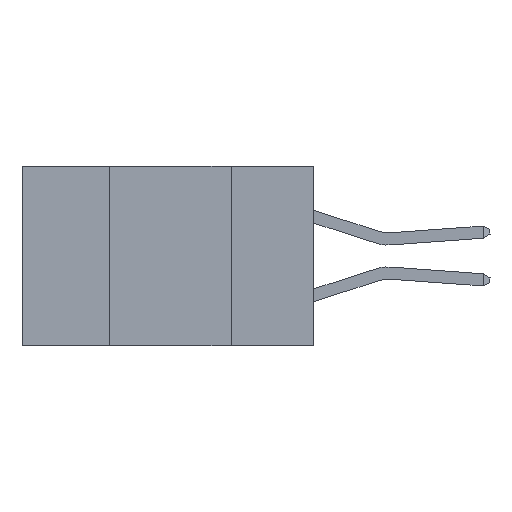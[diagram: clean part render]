
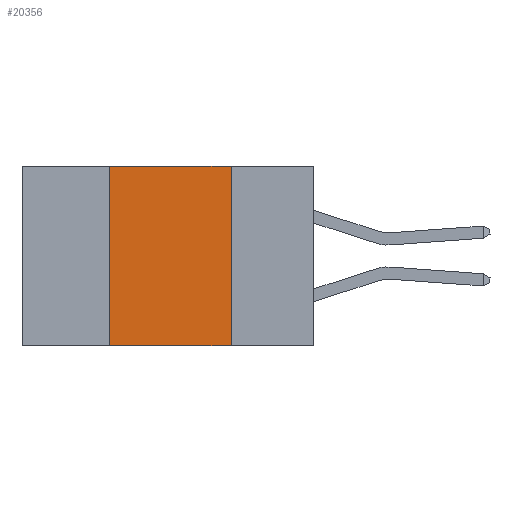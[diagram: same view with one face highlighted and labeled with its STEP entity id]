
A CAD part, left-side view. The second image highlights one B-rep face of the part: STEP entity #20356.
In plain terms, the highlighted planar face has unit normal (-1, 0, 0).
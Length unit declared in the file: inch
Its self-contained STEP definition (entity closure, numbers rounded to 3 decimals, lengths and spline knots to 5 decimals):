
#2487 = VECTOR ( 'NONE', #15811, 39.37008 ) ;
#3010 = VERTEX_POINT ( 'NONE', #18479 ) ;
#3021 = LINE ( 'NONE', #14083, #2487 ) ;
#4017 = LINE ( 'NONE', #10768, #20544 ) ;
#4413 = ORIENTED_EDGE ( 'NONE', *, *, #12895, .F. ) ;
#4940 = CARTESIAN_POINT ( 'NONE',  ( 0., 0.17, -0.37 ) ) ;
#5079 = CARTESIAN_POINT ( 'NONE',  ( 0., 0.6, 0. ) ) ;
#5647 = AXIS2_PLACEMENT_3D ( 'NONE', #5079, #17025, #6791 ) ;
#6791 = DIRECTION ( 'NONE',  ( 0., 0., -1. ) ) ;
#8664 = VERTEX_POINT ( 'NONE', #8680 ) ;
#8680 = CARTESIAN_POINT ( 'NONE',  ( 0., 0.42, 0. ) ) ;
#8958 = EDGE_CURVE ( 'NONE', #3010, #11951, #16744, .T. ) ;
#9199 = CARTESIAN_POINT ( 'NONE',  ( 0., 0.42, 0. ) ) ;
#10486 = FACE_OUTER_BOUND ( 'NONE', #15534, .T. ) ;
#10768 = CARTESIAN_POINT ( 'NONE',  ( 0., 0.6, 0. ) ) ;
#11546 = EDGE_CURVE ( 'NONE', #21383, #11951, #3021, .T. ) ;
#11951 = VERTEX_POINT ( 'NONE', #4940 ) ;
#12220 = VECTOR ( 'NONE', #19600, 39.37008 ) ;
#12268 = ORIENTED_EDGE ( 'NONE', *, *, #11546, .T. ) ;
#12567 = DIRECTION ( 'NONE',  ( 0., -1., 0. ) ) ;
#12895 = EDGE_CURVE ( 'NONE', #8664, #3010, #4017, .T. ) ;
#13022 = CARTESIAN_POINT ( 'NONE',  ( 0., 0.42, -0.37 ) ) ;
#14083 = CARTESIAN_POINT ( 'NONE',  ( 0., 0.6, -0.37 ) ) ;
#14125 = ORIENTED_EDGE ( 'NONE', *, *, #19923, .F. ) ;
#15534 = EDGE_LOOP ( 'NONE', ( #18294, #4413, #14125, #12268 ) ) ;
#15602 = VECTOR ( 'NONE', #21066, 39.37008 ) ;
#15811 = DIRECTION ( 'NONE',  ( 0., -1., 0. ) ) ;
#16132 = LINE ( 'NONE', #9199, #15602 ) ;
#16227 = CARTESIAN_POINT ( 'NONE',  ( 0., 0.17, 0. ) ) ;
#16744 = LINE ( 'NONE', #16227, #12220 ) ;
#17025 = DIRECTION ( 'NONE',  ( 1., 0., 0. ) ) ;
#18294 = ORIENTED_EDGE ( 'NONE', *, *, #8958, .F. ) ;
#18479 = CARTESIAN_POINT ( 'NONE',  ( 0., 0.17, 0. ) ) ;
#18649 = PLANE ( 'NONE',  #5647 ) ;
#19600 = DIRECTION ( 'NONE',  ( 0., 0., -1. ) ) ;
#19923 = EDGE_CURVE ( 'NONE', #21383, #8664, #16132, .T. ) ;
#20356 = ADVANCED_FACE ( 'NONE', ( #10486 ), #18649, .F. ) ;
#20544 = VECTOR ( 'NONE', #12567, 39.37008 ) ;
#21066 = DIRECTION ( 'NONE',  ( 0., 0., 1. ) ) ;
#21383 = VERTEX_POINT ( 'NONE', #13022 ) ;
